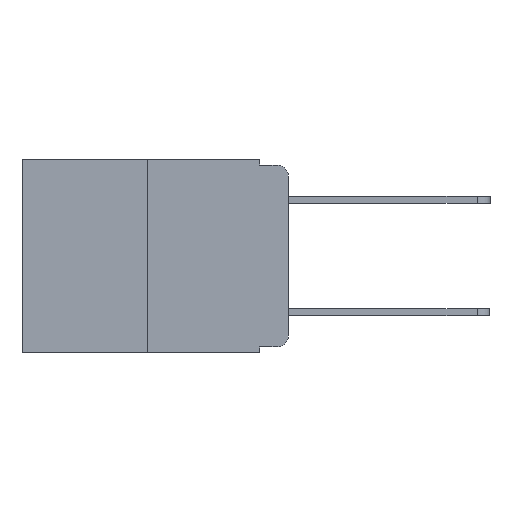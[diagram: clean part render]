
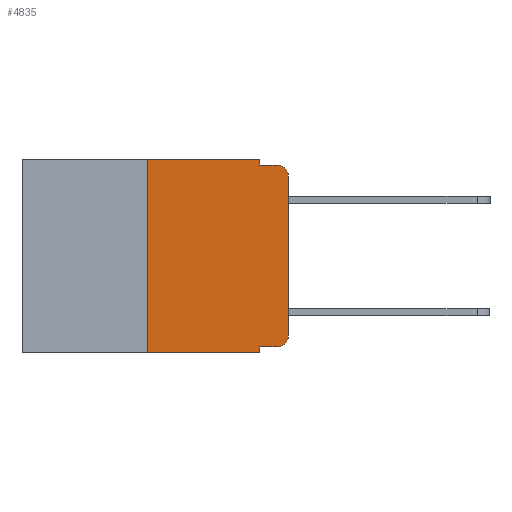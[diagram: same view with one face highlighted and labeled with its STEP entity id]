
A CAD part, left-side view. The second image highlights one B-rep face of the part: STEP entity #4835.
In plain terms, the highlighted planar face has unit normal (-1, 0, 0).
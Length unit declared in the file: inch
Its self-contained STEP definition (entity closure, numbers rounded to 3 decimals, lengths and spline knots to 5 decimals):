
#410 = CARTESIAN_POINT ( 'NONE',  ( 0., 0.02, -0.333 ) ) ;
#441 = LINE ( 'NONE', #16843, #13024 ) ;
#471 = ORIENTED_EDGE ( 'NONE', *, *, #9249, .F. ) ;
#678 = PLANE ( 'NONE',  #13397 ) ;
#1439 = VERTEX_POINT ( 'NONE', #18670 ) ;
#1540 = VECTOR ( 'NONE', #13768, 39.37008 ) ;
#2082 = LINE ( 'NONE', #4054, #1540 ) ;
#2161 = LINE ( 'NONE', #4136, #7150 ) ;
#2298 = VERTEX_POINT ( 'NONE', #410 ) ;
#2316 = CARTESIAN_POINT ( 'NONE',  ( 0., 0.473, -0.343 ) ) ;
#2625 = VERTEX_POINT ( 'NONE', #12964 ) ;
#2886 = CARTESIAN_POINT ( 'NONE',  ( 0., 0., -0.313 ) ) ;
#2937 = ORIENTED_EDGE ( 'NONE', *, *, #17875, .T. ) ;
#3266 = ORIENTED_EDGE ( 'NONE', *, *, #13858, .F. ) ;
#3335 = ORIENTED_EDGE ( 'NONE', *, *, #10126, .F. ) ;
#3600 = ORIENTED_EDGE ( 'NONE', *, *, #7175, .F. ) ;
#3654 = VERTEX_POINT ( 'NONE', #2886 ) ;
#3799 = EDGE_CURVE ( 'NONE', #1439, #10443, #13253, .T. ) ;
#3949 = ORIENTED_EDGE ( 'NONE', *, *, #8687, .T. ) ;
#3985 = ORIENTED_EDGE ( 'NONE', *, *, #3799, .F. ) ;
#3987 = DIRECTION ( 'NONE',  ( 0., -1., 0. ) ) ;
#4048 = VERTEX_POINT ( 'NONE', #13574 ) ;
#4054 = CARTESIAN_POINT ( 'NONE',  ( 0., 0.051, 0. ) ) ;
#4064 = DIRECTION ( 'NONE',  ( 1., 0., 0. ) ) ;
#4118 = VECTOR ( 'NONE', #8258, 39.37008 ) ;
#4131 = VECTOR ( 'NONE', #20258, 39.37008 ) ;
#4136 = CARTESIAN_POINT ( 'NONE',  ( 0., 0.473, 0. ) ) ;
#4422 = ORIENTED_EDGE ( 'NONE', *, *, #14116, .T. ) ;
#4536 = CIRCLE ( 'NONE', #17906, 0.02 ) ;
#4835 = ADVANCED_FACE ( 'NONE', ( #12716 ), #678, .F. ) ;
#5268 = VERTEX_POINT ( 'NONE', #17912 ) ;
#5280 = CARTESIAN_POINT ( 'NONE',  ( 0., 0.02, -0.01 ) ) ;
#5822 = DIRECTION ( 'NONE',  ( 0., -1., 0. ) ) ;
#6335 = DIRECTION ( 'NONE',  ( -1., 0., 0. ) ) ;
#6537 = ORIENTED_EDGE ( 'NONE', *, *, #16205, .T. ) ;
#6803 = CIRCLE ( 'NONE', #8796, 0.02 ) ;
#6891 = CARTESIAN_POINT ( 'NONE',  ( 0., 0.02, -0.03 ) ) ;
#7150 = VECTOR ( 'NONE', #5822, 39.37008 ) ;
#7175 = EDGE_CURVE ( 'NONE', #5268, #1439, #2082, .T. ) ;
#7191 = CARTESIAN_POINT ( 'NONE',  ( 0., 0., -0.03 ) ) ;
#7405 = CARTESIAN_POINT ( 'NONE',  ( 0., 0.051, 0. ) ) ;
#7424 = CARTESIAN_POINT ( 'NONE',  ( 0., 0.051, -0.343 ) ) ;
#7477 = VECTOR ( 'NONE', #16821, 39.37008 ) ;
#8258 = DIRECTION ( 'NONE',  ( 0., -1., 0. ) ) ;
#8551 = DIRECTION ( 'NONE',  ( 0., 0., -1. ) ) ;
#8684 = VERTEX_POINT ( 'NONE', #7424 ) ;
#8687 = EDGE_CURVE ( 'NONE', #3654, #14402, #17747, .T. ) ;
#8796 = AXIS2_PLACEMENT_3D ( 'NONE', #6891, #17823, #8551 ) ;
#9096 = DIRECTION ( 'NONE',  ( 0., 0., 1. ) ) ;
#9249 = EDGE_CURVE ( 'NONE', #4048, #8684, #19721, .T. ) ;
#9557 = VECTOR ( 'NONE', #9096, 39.37008 ) ;
#10126 = EDGE_CURVE ( 'NONE', #16742, #5268, #2161, .T. ) ;
#10443 = VERTEX_POINT ( 'NONE', #5280 ) ;
#10592 = CARTESIAN_POINT ( 'NONE',  ( 0., 0.473, 0. ) ) ;
#11278 = CARTESIAN_POINT ( 'NONE',  ( 0., 0.051, -0.333 ) ) ;
#11884 = EDGE_CURVE ( 'NONE', #14402, #10443, #6803, .T. ) ;
#12082 = CARTESIAN_POINT ( 'NONE',  ( 0., 0.25, 0. ) ) ;
#12248 = CARTESIAN_POINT ( 'NONE',  ( 0., 0., 0. ) ) ;
#12716 = FACE_OUTER_BOUND ( 'NONE', #15455, .T. ) ;
#12964 = CARTESIAN_POINT ( 'NONE',  ( 0., 0.25, -0.343 ) ) ;
#13024 = VECTOR ( 'NONE', #18285, 39.37008 ) ;
#13253 = LINE ( 'NONE', #14551, #4118 ) ;
#13397 = AXIS2_PLACEMENT_3D ( 'NONE', #10592, #4064, #15325 ) ;
#13574 = CARTESIAN_POINT ( 'NONE',  ( 0., 0.051, -0.333 ) ) ;
#13768 = DIRECTION ( 'NONE',  ( 0., 0., -1. ) ) ;
#13858 = EDGE_CURVE ( 'NONE', #2625, #16742, #441, .T. ) ;
#14116 = EDGE_CURVE ( 'NONE', #4048, #2298, #19775, .T. ) ;
#14402 = VERTEX_POINT ( 'NONE', #7191 ) ;
#14551 = CARTESIAN_POINT ( 'NONE',  ( 0., 0.051, -0.01 ) ) ;
#14795 = ORIENTED_EDGE ( 'NONE', *, *, #11884, .T. ) ;
#15325 = DIRECTION ( 'NONE',  ( 0., 0., -1. ) ) ;
#15455 = EDGE_LOOP ( 'NONE', ( #3949, #14795, #3985, #3600, #3335, #3266, #2937, #471, #4422, #6537 ) ) ;
#15845 = CARTESIAN_POINT ( 'NONE',  ( 0., 0.02, -0.313 ) ) ;
#16205 = EDGE_CURVE ( 'NONE', #2298, #3654, #4536, .T. ) ;
#16742 = VERTEX_POINT ( 'NONE', #12082 ) ;
#16821 = DIRECTION ( 'NONE',  ( 0., 0., -1. ) ) ;
#16843 = CARTESIAN_POINT ( 'NONE',  ( 0., 0.25, 0. ) ) ;
#17330 = DIRECTION ( 'NONE',  ( 0., 0., -1. ) ) ;
#17747 = LINE ( 'NONE', #12248, #9557 ) ;
#17823 = DIRECTION ( 'NONE',  ( -1., 0., 0. ) ) ;
#17875 = EDGE_CURVE ( 'NONE', #2625, #8684, #19649, .T. ) ;
#17906 = AXIS2_PLACEMENT_3D ( 'NONE', #15845, #6335, #17330 ) ;
#17912 = CARTESIAN_POINT ( 'NONE',  ( 0., 0.051, 0. ) ) ;
#18285 = DIRECTION ( 'NONE',  ( 0., 0., 1. ) ) ;
#18670 = CARTESIAN_POINT ( 'NONE',  ( 0., 0.051, -0.01 ) ) ;
#19206 = VECTOR ( 'NONE', #3987, 39.37008 ) ;
#19649 = LINE ( 'NONE', #2316, #19206 ) ;
#19721 = LINE ( 'NONE', #7405, #7477 ) ;
#19775 = LINE ( 'NONE', #11278, #4131 ) ;
#20258 = DIRECTION ( 'NONE',  ( 0., -1., 0. ) ) ;
